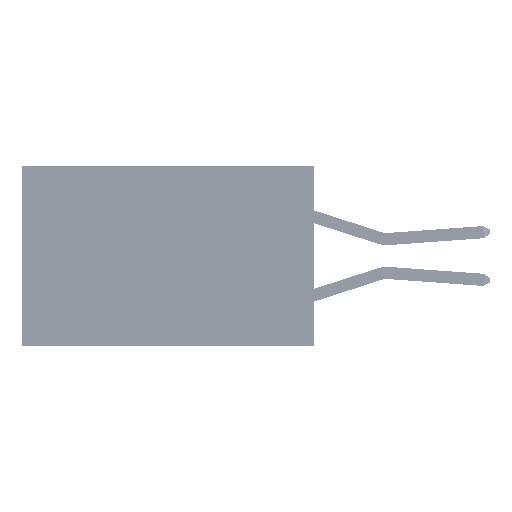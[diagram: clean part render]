
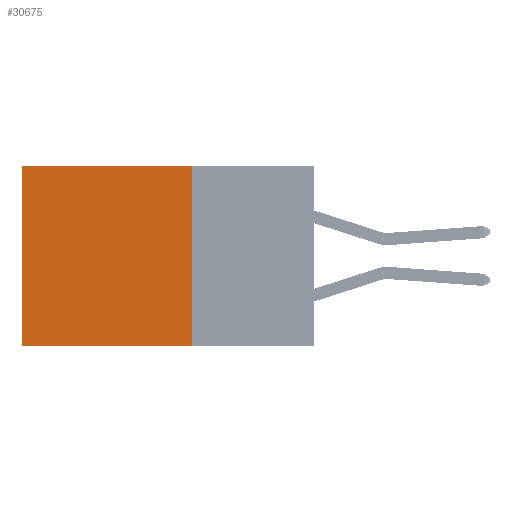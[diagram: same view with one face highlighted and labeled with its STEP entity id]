
A CAD part, left-side view. The second image highlights one B-rep face of the part: STEP entity #30675.
In plain terms, the highlighted planar face has unit normal (-1, 0, 0).
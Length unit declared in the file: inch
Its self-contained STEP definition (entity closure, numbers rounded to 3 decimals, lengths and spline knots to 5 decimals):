
#913 = DIRECTION ( 'NONE',  ( 0., 0., -1. ) ) ;
#1646 = CARTESIAN_POINT ( 'NONE',  ( 0.2875, 0.25, -0.37 ) ) ;
#2343 = ORIENTED_EDGE ( 'NONE', *, *, #32615, .T. ) ;
#6909 = EDGE_CURVE ( 'NONE', #18547, #31216, #50402, .T. ) ;
#7043 = VERTEX_POINT ( 'NONE', #39601 ) ;
#9869 = DIRECTION ( 'NONE',  ( 0., 0., -1. ) ) ;
#13317 = CARTESIAN_POINT ( 'NONE',  ( 0.2875, 0.25, 0. ) ) ;
#13333 = DIRECTION ( 'NONE',  ( 0., 1., 0. ) ) ;
#15310 = CARTESIAN_POINT ( 'NONE',  ( 0.2875, 0.25, -0.37 ) ) ;
#15377 = VECTOR ( 'NONE', #13333, 39.37008 ) ;
#15966 = LINE ( 'NONE', #31764, #47734 ) ;
#16373 = LINE ( 'NONE', #13317, #27422 ) ;
#18547 = VERTEX_POINT ( 'NONE', #15310 ) ;
#20837 = AXIS2_PLACEMENT_3D ( 'NONE', #51225, #42902, #9869 ) ;
#22510 = LINE ( 'NONE', #52621, #36076 ) ;
#27422 = VECTOR ( 'NONE', #913, 39.37008 ) ;
#28157 = ORIENTED_EDGE ( 'NONE', *, *, #6909, .F. ) ;
#29274 = VERTEX_POINT ( 'NONE', #53415 ) ;
#30675 = ADVANCED_FACE ( 'NONE', ( #46620 ), #42565, .F. ) ;
#31216 = VERTEX_POINT ( 'NONE', #37991 ) ;
#31585 = DIRECTION ( 'NONE',  ( 0., 0., -1. ) ) ;
#31764 = CARTESIAN_POINT ( 'NONE',  ( 0.2875, 0.6, 0. ) ) ;
#32615 = EDGE_CURVE ( 'NONE', #29274, #7043, #22510, .T. ) ;
#33257 = EDGE_CURVE ( 'NONE', #7043, #31216, #15966, .T. ) ;
#33694 = ORIENTED_EDGE ( 'NONE', *, *, #38784, .F. ) ;
#34465 = EDGE_LOOP ( 'NONE', ( #39199, #28157, #33694, #2343 ) ) ;
#36076 = VECTOR ( 'NONE', #40334, 39.37008 ) ;
#37991 = CARTESIAN_POINT ( 'NONE',  ( 0.2875, 0.6, -0.37 ) ) ;
#38784 = EDGE_CURVE ( 'NONE', #29274, #18547, #16373, .T. ) ;
#39199 = ORIENTED_EDGE ( 'NONE', *, *, #33257, .T. ) ;
#39601 = CARTESIAN_POINT ( 'NONE',  ( 0.2875, 0.6, 0. ) ) ;
#40334 = DIRECTION ( 'NONE',  ( 0., 1., 0. ) ) ;
#42565 = PLANE ( 'NONE',  #20837 ) ;
#42902 = DIRECTION ( 'NONE',  ( 1., 0., 0. ) ) ;
#46620 = FACE_OUTER_BOUND ( 'NONE', #34465, .T. ) ;
#47734 = VECTOR ( 'NONE', #31585, 39.37008 ) ;
#50402 = LINE ( 'NONE', #1646, #15377 ) ;
#51225 = CARTESIAN_POINT ( 'NONE',  ( 0.2875, 0.25, 0. ) ) ;
#52621 = CARTESIAN_POINT ( 'NONE',  ( 0.2875, 0.25, 0. ) ) ;
#53415 = CARTESIAN_POINT ( 'NONE',  ( 0.2875, 0.25, 0. ) ) ;
